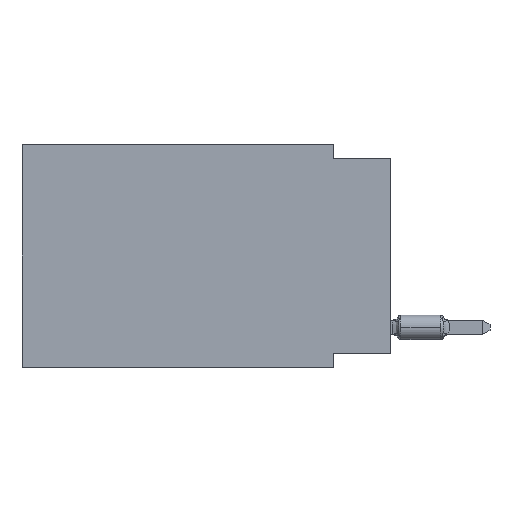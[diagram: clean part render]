
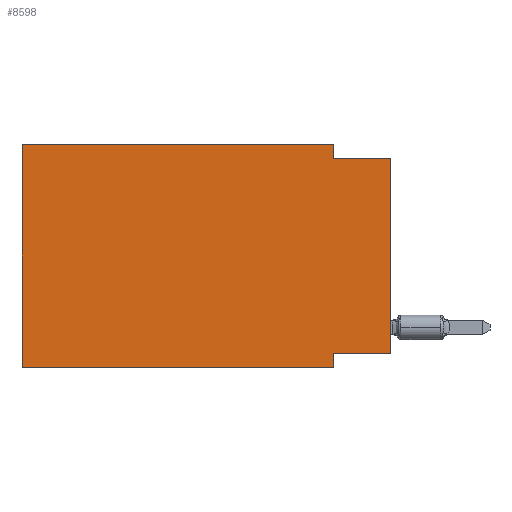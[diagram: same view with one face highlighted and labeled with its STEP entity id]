
A CAD part, left-side view. The second image highlights one B-rep face of the part: STEP entity #8598.
In plain terms, the highlighted planar face has unit normal (-1, 0, 0).
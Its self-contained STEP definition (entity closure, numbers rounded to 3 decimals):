
#17 = DIRECTION ( 'NONE',  ( 0., 0., 1. ) ) ;
#342 = EDGE_CURVE ( 'NONE', #2295, #4944, #13065, .T. ) ;
#431 = CARTESIAN_POINT ( 'NONE',  ( 0., 16.383, 0. ) ) ;
#585 = VERTEX_POINT ( 'NONE', #3148 ) ;
#919 = VERTEX_POINT ( 'NONE', #7451 ) ;
#1343 = DIRECTION ( 'NONE',  ( 0., -1., 0. ) ) ;
#1367 = VERTEX_POINT ( 'NONE', #1636 ) ;
#1489 = PLANE ( 'NONE',  #12369 ) ;
#1636 = CARTESIAN_POINT ( 'NONE',  ( 0., 0., -9.271 ) ) ;
#1680 = CARTESIAN_POINT ( 'NONE',  ( 0., 2.54, -9.271 ) ) ;
#1898 = VECTOR ( 'NONE', #5144, 1000. ) ;
#2145 = DIRECTION ( 'NONE',  ( 0., -1., 0. ) ) ;
#2295 = VERTEX_POINT ( 'NONE', #1680 ) ;
#2741 = DIRECTION ( 'NONE',  ( 0., 0., -1. ) ) ;
#2745 = ORIENTED_EDGE ( 'NONE', *, *, #7999, .T. ) ;
#2869 = VECTOR ( 'NONE', #13360, 1000. ) ;
#3148 = CARTESIAN_POINT ( 'NONE',  ( 0., 16.383, -9.906 ) ) ;
#3543 = ORIENTED_EDGE ( 'NONE', *, *, #6876, .F. ) ;
#3851 = EDGE_CURVE ( 'NONE', #585, #12926, #11276, .T. ) ;
#4496 = LINE ( 'NONE', #13300, #15181 ) ;
#4573 = EDGE_CURVE ( 'NONE', #12926, #15440, #13274, .T. ) ;
#4788 = CARTESIAN_POINT ( 'NONE',  ( 0., 0., -0.635 ) ) ;
#4944 = VERTEX_POINT ( 'NONE', #15470 ) ;
#5144 = DIRECTION ( 'NONE',  ( 0., 0., 1. ) ) ;
#5192 = ORIENTED_EDGE ( 'NONE', *, *, #9205, .T. ) ;
#5892 = VECTOR ( 'NONE', #17, 1000. ) ;
#6410 = CARTESIAN_POINT ( 'NONE',  ( 0., 16.383, 0. ) ) ;
#6423 = VERTEX_POINT ( 'NONE', #11812 ) ;
#6859 = VECTOR ( 'NONE', #1343, 1000. ) ;
#6876 = EDGE_CURVE ( 'NONE', #1367, #2295, #4496, .T. ) ;
#7020 = DIRECTION ( 'NONE',  ( 0., 0., -1. ) ) ;
#7317 = DIRECTION ( 'NONE',  ( 0., 1., 0. ) ) ;
#7451 = CARTESIAN_POINT ( 'NONE',  ( 0., 0., -0.635 ) ) ;
#7454 = FACE_OUTER_BOUND ( 'NONE', #8765, .T. ) ;
#7999 = EDGE_CURVE ( 'NONE', #585, #4944, #9212, .T. ) ;
#8125 = VECTOR ( 'NONE', #2741, 1000. ) ;
#8558 = VECTOR ( 'NONE', #7020, 1000. ) ;
#8598 = ADVANCED_FACE ( 'NONE', ( #7454 ), #1489, .F. ) ;
#8765 = EDGE_LOOP ( 'NONE', ( #5192, #14580, #8843, #13106, #9095, #2745, #11753, #3543 ) ) ;
#8780 = LINE ( 'NONE', #14695, #8125 ) ;
#8843 = ORIENTED_EDGE ( 'NONE', *, *, #13732, .F. ) ;
#9095 = ORIENTED_EDGE ( 'NONE', *, *, #3851, .F. ) ;
#9152 = CARTESIAN_POINT ( 'NONE',  ( 0., 2.54, -9.906 ) ) ;
#9205 = EDGE_CURVE ( 'NONE', #1367, #919, #14393, .T. ) ;
#9212 = LINE ( 'NONE', #13998, #10067 ) ;
#10067 = VECTOR ( 'NONE', #2145, 1000. ) ;
#10534 = CARTESIAN_POINT ( 'NONE',  ( 0., 16.383, 0. ) ) ;
#11151 = DIRECTION ( 'NONE',  ( 0., 0., -1. ) ) ;
#11276 = LINE ( 'NONE', #6410, #1898 ) ;
#11753 = ORIENTED_EDGE ( 'NONE', *, *, #342, .F. ) ;
#11812 = CARTESIAN_POINT ( 'NONE',  ( 0., 2.54, -0.635 ) ) ;
#12015 = CARTESIAN_POINT ( 'NONE',  ( 0., 0., 0. ) ) ;
#12369 = AXIS2_PLACEMENT_3D ( 'NONE', #14770, #13591, #11151 ) ;
#12926 = VERTEX_POINT ( 'NONE', #431 ) ;
#13065 = LINE ( 'NONE', #9152, #8558 ) ;
#13106 = ORIENTED_EDGE ( 'NONE', *, *, #4573, .F. ) ;
#13161 = EDGE_CURVE ( 'NONE', #6423, #919, #13284, .T. ) ;
#13274 = LINE ( 'NONE', #10534, #6859 ) ;
#13284 = LINE ( 'NONE', #4788, #2869 ) ;
#13300 = CARTESIAN_POINT ( 'NONE',  ( 0., 0., -9.271 ) ) ;
#13360 = DIRECTION ( 'NONE',  ( 0., -1., 0. ) ) ;
#13591 = DIRECTION ( 'NONE',  ( 1., 0., 0. ) ) ;
#13732 = EDGE_CURVE ( 'NONE', #15440, #6423, #8780, .T. ) ;
#13998 = CARTESIAN_POINT ( 'NONE',  ( 0., 16.383, -9.906 ) ) ;
#14393 = LINE ( 'NONE', #12015, #5892 ) ;
#14580 = ORIENTED_EDGE ( 'NONE', *, *, #13161, .F. ) ;
#14695 = CARTESIAN_POINT ( 'NONE',  ( 0., 2.54, 0. ) ) ;
#14752 = CARTESIAN_POINT ( 'NONE',  ( 0., 2.54, 0. ) ) ;
#14770 = CARTESIAN_POINT ( 'NONE',  ( 0., 16.383, 0. ) ) ;
#15181 = VECTOR ( 'NONE', #7317, 1000. ) ;
#15440 = VERTEX_POINT ( 'NONE', #14752 ) ;
#15470 = CARTESIAN_POINT ( 'NONE',  ( 0., 2.54, -9.906 ) ) ;
